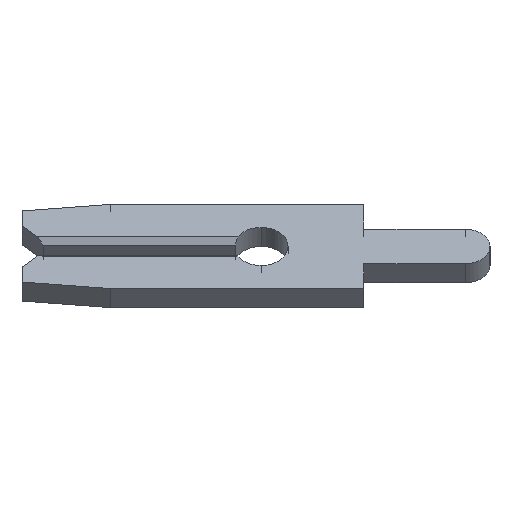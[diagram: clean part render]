
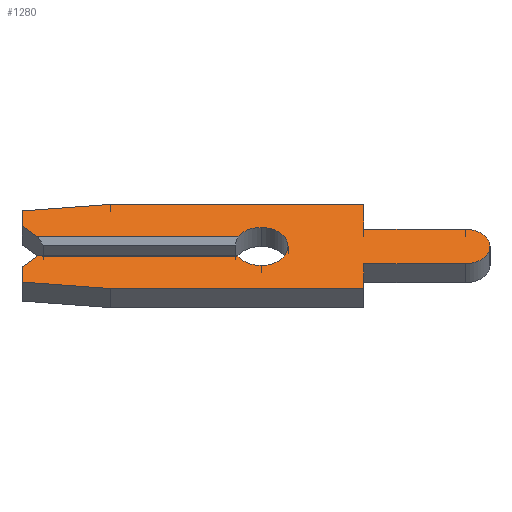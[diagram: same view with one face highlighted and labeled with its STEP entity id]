
A CAD part, left-side view. The second image highlights one B-rep face of the part: STEP entity #1280.
In plain terms, the highlighted face is planar.
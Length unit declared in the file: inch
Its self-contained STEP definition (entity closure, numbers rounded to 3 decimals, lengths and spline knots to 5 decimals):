
#4 = LINE ( 'NONE', #1057, #243 ) ;
#6 = VERTEX_POINT ( 'NONE', #685 ) ;
#20 = ORIENTED_EDGE ( 'NONE', *, *, #143, .F. ) ;
#33 = EDGE_CURVE ( 'NONE', #1522, #401, #574, .T. ) ;
#50 = CARTESIAN_POINT ( 'NONE',  ( -0.013, 0., 0. ) ) ;
#56 = DIRECTION ( 'NONE',  ( 0., 0., -1. ) ) ;
#70 = PLANE ( 'NONE',  #650 ) ;
#74 = AXIS2_PLACEMENT_3D ( 'NONE', #139, #128, #237 ) ;
#79 = VECTOR ( 'NONE', #1020, 39.37008 ) ;
#82 = EDGE_CURVE ( 'NONE', #361, #1278, #432, .T. ) ;
#102 = DIRECTION ( 'NONE',  ( -1., 0., 0. ) ) ;
#108 = CARTESIAN_POINT ( 'NONE',  ( -0.013, -0.099, 0.0575 ) ) ;
#128 = DIRECTION ( 'NONE',  ( -1., 0., 0. ) ) ;
#139 = CARTESIAN_POINT ( 'NONE',  ( -0.013, 0., 0. ) ) ;
#143 = EDGE_CURVE ( 'NONE', #1542, #526, #4, .T. ) ;
#157 = CARTESIAN_POINT ( 'NONE',  ( -0.013, -0.099, 0.0235 ) ) ;
#161 = CARTESIAN_POINT ( 'NONE',  ( -0.013, -0.099, -0.0235 ) ) ;
#166 = CARTESIAN_POINT ( 'NONE',  ( -0.013, 0.2105, -0.0075 ) ) ;
#175 = CIRCLE ( 'NONE', #1132, 0.026 ) ;
#183 = VERTEX_POINT ( 'NONE', #943 ) ;
#184 = AXIS2_PLACEMENT_3D ( 'NONE', #1038, #1175, #449 ) ;
#212 = CARTESIAN_POINT ( 'NONE',  ( -0.013, -0.1975, 0.0235 ) ) ;
#221 = EDGE_CURVE ( 'NONE', #1211, #6, #576, .T. ) ;
#237 = DIRECTION ( 'NONE',  ( 0., 0., -1. ) ) ;
#242 = EDGE_CURVE ( 'NONE', #1023, #1522, #358, .T. ) ;
#243 = VECTOR ( 'NONE', #350, 39.37008 ) ;
#247 = ORIENTED_EDGE ( 'NONE', *, *, #1143, .T. ) ;
#249 = CARTESIAN_POINT ( 'NONE',  ( -0.013, 0.146, 0.0575 ) ) ;
#254 = ORIENTED_EDGE ( 'NONE', *, *, #1037, .F. ) ;
#257 = CARTESIAN_POINT ( 'NONE',  ( -0.013, 0.231, 0.028 ) ) ;
#278 = DIRECTION ( 'NONE',  ( 0., 1., 0. ) ) ;
#281 = ORIENTED_EDGE ( 'NONE', *, *, #464, .F. ) ;
#286 = CARTESIAN_POINT ( 'NONE',  ( -0.013, 0.216, -0.013 ) ) ;
#296 = DIRECTION ( 'NONE',  ( 0., -1., 0. ) ) ;
#297 = ORIENTED_EDGE ( 'NONE', *, *, #1452, .F. ) ;
#307 = CARTESIAN_POINT ( 'NONE',  ( -0.013, 0.146, -0.0575 ) ) ;
#328 = EDGE_CURVE ( 'NONE', #1311, #1151, #1446, .T. ) ;
#338 = DIRECTION ( 'NONE',  ( 0., 0., 1. ) ) ;
#350 = DIRECTION ( 'NONE',  ( 0., 0., -1. ) ) ;
#358 = LINE ( 'NONE', #1034, #438 ) ;
#361 = VERTEX_POINT ( 'NONE', #212 ) ;
#365 = LINE ( 'NONE', #166, #79 ) ;
#401 = VERTEX_POINT ( 'NONE', #1291 ) ;
#432 = CIRCLE ( 'NONE', #184, 0.0235 ) ;
#438 = VECTOR ( 'NONE', #1395, 39.37008 ) ;
#439 = LINE ( 'NONE', #1325, #468 ) ;
#442 = ORIENTED_EDGE ( 'NONE', *, *, #1477, .F. ) ;
#444 = CARTESIAN_POINT ( 'NONE',  ( -0.013, 0.231, 0.04857 ) ) ;
#448 = CIRCLE ( 'NONE', #74, 0.026 ) ;
#449 = DIRECTION ( 'NONE',  ( 0., 0., 1. ) ) ;
#464 = EDGE_CURVE ( 'NONE', #183, #1518, #448, .T. ) ;
#468 = VECTOR ( 'NONE', #1299, 39.37008 ) ;
#474 = CARTESIAN_POINT ( 'NONE',  ( -0.013, -0.099, -0.0575 ) ) ;
#483 = VECTOR ( 'NONE', #338, 39.37008 ) ;
#488 = FACE_OUTER_BOUND ( 'NONE', #1471, .T. ) ;
#504 = LINE ( 'NONE', #307, #1348 ) ;
#526 = VERTEX_POINT ( 'NONE', #611 ) ;
#529 = ORIENTED_EDGE ( 'NONE', *, *, #33, .F. ) ;
#574 = LINE ( 'NONE', #444, #1358 ) ;
#576 = LINE ( 'NONE', #1071, #737 ) ;
#584 = CARTESIAN_POINT ( 'NONE',  ( -0.013, -0.1975, -0.0235 ) ) ;
#590 = DIRECTION ( 'NONE',  ( 0., 0., -1. ) ) ;
#603 = CARTESIAN_POINT ( 'NONE',  ( -0.013, 0.231, -0.028 ) ) ;
#608 = ORIENTED_EDGE ( 'NONE', *, *, #242, .F. ) ;
#611 = CARTESIAN_POINT ( 'NONE',  ( -0.013, -0.099, 0.0235 ) ) ;
#650 = AXIS2_PLACEMENT_3D ( 'NONE', #1046, #1055, #1284 ) ;
#667 = EDGE_CURVE ( 'NONE', #401, #1542, #1224, .T. ) ;
#674 = ORIENTED_EDGE ( 'NONE', *, *, #908, .F. ) ;
#677 = LINE ( 'NONE', #161, #1271 ) ;
#685 = CARTESIAN_POINT ( 'NONE',  ( -0.013, 0.02252, -0.013 ) ) ;
#697 = CARTESIAN_POINT ( 'NONE',  ( -0.013, 0.146, -0.0575 ) ) ;
#737 = VECTOR ( 'NONE', #1544, 39.37008 ) ;
#749 = ORIENTED_EDGE ( 'NONE', *, *, #1437, .F. ) ;
#772 = DIRECTION ( 'NONE',  ( 0., -1., 0. ) ) ;
#797 = LINE ( 'NONE', #1265, #955 ) ;
#817 = CIRCLE ( 'NONE', #1490, 0.026 ) ;
#823 = CARTESIAN_POINT ( 'NONE',  ( -0.013, 0.02252, 0.013 ) ) ;
#834 = ORIENTED_EDGE ( 'NONE', *, *, #1403, .F. ) ;
#852 = CARTESIAN_POINT ( 'NONE',  ( -0.013, 0.2105, 0.0075 ) ) ;
#857 = CARTESIAN_POINT ( 'NONE',  ( -0.013, 0., 0. ) ) ;
#899 = ORIENTED_EDGE ( 'NONE', *, *, #1032, .F. ) ;
#900 = VECTOR ( 'NONE', #1461, 39.37008 ) ;
#908 = EDGE_CURVE ( 'NONE', #526, #361, #1169, .T. ) ;
#943 = CARTESIAN_POINT ( 'NONE',  ( -0.013, 0., 0.026 ) ) ;
#955 = VECTOR ( 'NONE', #296, 39.37008 ) ;
#961 = ORIENTED_EDGE ( 'NONE', *, *, #667, .F. ) ;
#994 = ORIENTED_EDGE ( 'NONE', *, *, #82, .F. ) ;
#1020 = DIRECTION ( 'NONE',  ( 0., -0.707, 0.707 ) ) ;
#1023 = VERTEX_POINT ( 'NONE', #257 ) ;
#1029 = DIRECTION ( 'NONE',  ( -1., 0., 0. ) ) ;
#1032 = EDGE_CURVE ( 'NONE', #1278, #1077, #677, .T. ) ;
#1034 = CARTESIAN_POINT ( 'NONE',  ( -0.013, 0.231, 0.028 ) ) ;
#1037 = EDGE_CURVE ( 'NONE', #6, #1394, #175, .T. ) ;
#1038 = CARTESIAN_POINT ( 'NONE',  ( -0.013, -0.1975, 0. ) ) ;
#1046 = CARTESIAN_POINT ( 'NONE',  ( -0.013, 0., 0. ) ) ;
#1047 = VECTOR ( 'NONE', #772, 39.37008 ) ;
#1055 = DIRECTION ( 'NONE',  ( 1., 0., 0. ) ) ;
#1057 = CARTESIAN_POINT ( 'NONE',  ( -0.013, -0.099, 0.0575 ) ) ;
#1068 = CARTESIAN_POINT ( 'NONE',  ( -0.013, 0.231, -0.04857 ) ) ;
#1071 = CARTESIAN_POINT ( 'NONE',  ( -0.013, 0., -0.013 ) ) ;
#1077 = VERTEX_POINT ( 'NONE', #1372 ) ;
#1132 = AXIS2_PLACEMENT_3D ( 'NONE', #50, #1029, #56 ) ;
#1139 = CARTESIAN_POINT ( 'NONE',  ( -0.013, 0.231, -0.028 ) ) ;
#1143 = EDGE_CURVE ( 'NONE', #1174, #1518, #797, .T. ) ;
#1151 = VERTEX_POINT ( 'NONE', #1139 ) ;
#1156 = ORIENTED_EDGE ( 'NONE', *, *, #328, .F. ) ;
#1167 = LINE ( 'NONE', #852, #1486 ) ;
#1169 = LINE ( 'NONE', #157, #1047 ) ;
#1171 = DIRECTION ( 'NONE',  ( 0., 1., 0. ) ) ;
#1174 = VERTEX_POINT ( 'NONE', #1502 ) ;
#1175 = DIRECTION ( 'NONE',  ( 1., 0., 0. ) ) ;
#1185 = CARTESIAN_POINT ( 'NONE',  ( -0.013, 0.231, -0.04857 ) ) ;
#1207 = EDGE_CURVE ( 'NONE', #1151, #1211, #365, .T. ) ;
#1211 = VERTEX_POINT ( 'NONE', #286 ) ;
#1224 = LINE ( 'NONE', #249, #900 ) ;
#1234 = ORIENTED_EDGE ( 'NONE', *, *, #221, .F. ) ;
#1247 = ORIENTED_EDGE ( 'NONE', *, *, #1207, .F. ) ;
#1265 = CARTESIAN_POINT ( 'NONE',  ( -0.013, 0.231, 0.013 ) ) ;
#1271 = VECTOR ( 'NONE', #278, 39.37008 ) ;
#1278 = VERTEX_POINT ( 'NONE', #584 ) ;
#1280 = ADVANCED_FACE ( 'NONE', ( #488 ), #70, .F. ) ;
#1284 = DIRECTION ( 'NONE',  ( 0., 0., -1. ) ) ;
#1291 = CARTESIAN_POINT ( 'NONE',  ( -0.013, 0.146, 0.0575 ) ) ;
#1299 = DIRECTION ( 'NONE',  ( 0., 0., -1. ) ) ;
#1305 = EDGE_CURVE ( 'NONE', #1496, #1314, #504, .T. ) ;
#1310 = DIRECTION ( 'NONE',  ( 0., 0.707, 0.707 ) ) ;
#1311 = VERTEX_POINT ( 'NONE', #1185 ) ;
#1314 = VERTEX_POINT ( 'NONE', #697 ) ;
#1323 = CARTESIAN_POINT ( 'NONE',  ( -0.013, 0.231, 0.04857 ) ) ;
#1325 = CARTESIAN_POINT ( 'NONE',  ( -0.013, -0.099, -0.0575 ) ) ;
#1348 = VECTOR ( 'NONE', #1171, 39.37008 ) ;
#1351 = ORIENTED_EDGE ( 'NONE', *, *, #1305, .F. ) ;
#1358 = VECTOR ( 'NONE', #1390, 39.37008 ) ;
#1372 = CARTESIAN_POINT ( 'NONE',  ( -0.013, -0.099, -0.0235 ) ) ;
#1390 = DIRECTION ( 'NONE',  ( 0., -0.995, 0.105 ) ) ;
#1394 = VERTEX_POINT ( 'NONE', #1443 ) ;
#1395 = DIRECTION ( 'NONE',  ( 0., 0., 1. ) ) ;
#1403 = EDGE_CURVE ( 'NONE', #1077, #1496, #439, .T. ) ;
#1427 = DIRECTION ( 'NONE',  ( 0., 0.995, 0.105 ) ) ;
#1437 = EDGE_CURVE ( 'NONE', #1394, #183, #817, .T. ) ;
#1443 = CARTESIAN_POINT ( 'NONE',  ( -0.013, 0., -0.026 ) ) ;
#1446 = LINE ( 'NONE', #603, #483 ) ;
#1451 = LINE ( 'NONE', #1068, #1472 ) ;
#1452 = EDGE_CURVE ( 'NONE', #1314, #1311, #1451, .T. ) ;
#1461 = DIRECTION ( 'NONE',  ( 0., -1., 0. ) ) ;
#1471 = EDGE_LOOP ( 'NONE', ( #247, #281, #749, #254, #1234, #1247, #1156, #297, #1351, #834, #899, #994, #674, #20, #961, #529, #608, #442 ) ) ;
#1472 = VECTOR ( 'NONE', #1427, 39.37008 ) ;
#1477 = EDGE_CURVE ( 'NONE', #1174, #1023, #1167, .T. ) ;
#1486 = VECTOR ( 'NONE', #1310, 39.37008 ) ;
#1490 = AXIS2_PLACEMENT_3D ( 'NONE', #857, #102, #590 ) ;
#1496 = VERTEX_POINT ( 'NONE', #474 ) ;
#1502 = CARTESIAN_POINT ( 'NONE',  ( -0.013, 0.216, 0.013 ) ) ;
#1518 = VERTEX_POINT ( 'NONE', #823 ) ;
#1522 = VERTEX_POINT ( 'NONE', #1323 ) ;
#1542 = VERTEX_POINT ( 'NONE', #108 ) ;
#1544 = DIRECTION ( 'NONE',  ( 0., -1., 0. ) ) ;
